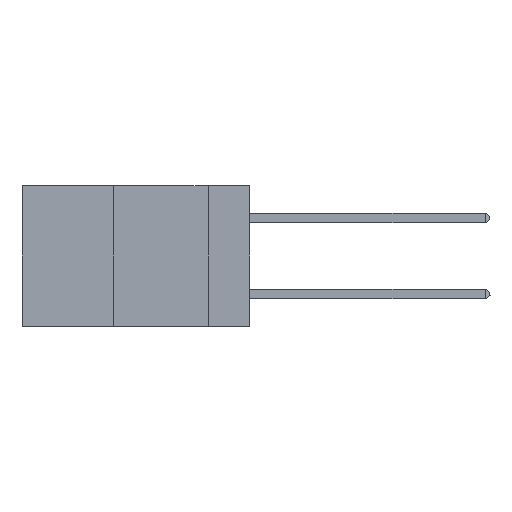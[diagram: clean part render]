
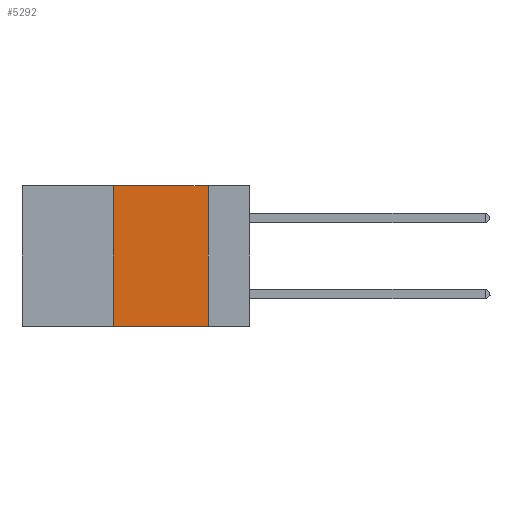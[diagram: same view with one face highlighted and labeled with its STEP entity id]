
A CAD part, left-side view. The second image highlights one B-rep face of the part: STEP entity #5292.
In plain terms, the highlighted planar face has unit normal (-1, 0, 0).
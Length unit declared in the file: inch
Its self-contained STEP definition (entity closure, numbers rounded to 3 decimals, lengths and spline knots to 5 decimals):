
#268 = CARTESIAN_POINT ( 'NONE',  ( 0., 0.36, 0. ) ) ;
#1010 = LINE ( 'NONE', #16282, #7445 ) ;
#1446 = VECTOR ( 'NONE', #27344, 39.37008 ) ;
#1500 = EDGE_CURVE ( 'NONE', #24219, #27783, #1010, .T. ) ;
#2094 = LINE ( 'NONE', #18200, #26129 ) ;
#2133 = CARTESIAN_POINT ( 'NONE',  ( 0., 0.36, 0. ) ) ;
#3128 = ORIENTED_EDGE ( 'NONE', *, *, #10522, .F. ) ;
#5292 = ADVANCED_FACE ( 'NONE', ( #23066 ), #11940, .F. ) ;
#7445 = VECTOR ( 'NONE', #11656, 39.37008 ) ;
#9451 = LINE ( 'NONE', #2133, #1446 ) ;
#10522 = EDGE_CURVE ( 'NONE', #24219, #12321, #9451, .T. ) ;
#11181 = VERTEX_POINT ( 'NONE', #14062 ) ;
#11422 = EDGE_LOOP ( 'NONE', ( #26074, #19471, #3128, #15519 ) ) ;
#11656 = DIRECTION ( 'NONE',  ( 0., -1., 0. ) ) ;
#11940 = PLANE ( 'NONE',  #20525 ) ;
#12321 = VERTEX_POINT ( 'NONE', #268 ) ;
#14044 = VECTOR ( 'NONE', #17275, 39.37008 ) ;
#14062 = CARTESIAN_POINT ( 'NONE',  ( 0., 0.11, 0. ) ) ;
#14481 = DIRECTION ( 'NONE',  ( 0., 0., -1. ) ) ;
#14801 = CARTESIAN_POINT ( 'NONE',  ( 0., 0.6, 0. ) ) ;
#15295 = CARTESIAN_POINT ( 'NONE',  ( 0., 0.11, -0.37 ) ) ;
#15519 = ORIENTED_EDGE ( 'NONE', *, *, #1500, .T. ) ;
#16282 = CARTESIAN_POINT ( 'NONE',  ( 0., 0.6, -0.37 ) ) ;
#17275 = DIRECTION ( 'NONE',  ( 0., -1., 0. ) ) ;
#18200 = CARTESIAN_POINT ( 'NONE',  ( 0., 0.11, 0. ) ) ;
#19471 = ORIENTED_EDGE ( 'NONE', *, *, #24892, .F. ) ;
#20525 = AXIS2_PLACEMENT_3D ( 'NONE', #14801, #29827, #14481 ) ;
#20664 = DIRECTION ( 'NONE',  ( 0., 0., -1. ) ) ;
#23066 = FACE_OUTER_BOUND ( 'NONE', #11422, .T. ) ;
#24219 = VERTEX_POINT ( 'NONE', #32777 ) ;
#24472 = EDGE_CURVE ( 'NONE', #11181, #27783, #2094, .T. ) ;
#24892 = EDGE_CURVE ( 'NONE', #12321, #11181, #27717, .T. ) ;
#25260 = CARTESIAN_POINT ( 'NONE',  ( 0., 0.6, 0. ) ) ;
#26074 = ORIENTED_EDGE ( 'NONE', *, *, #24472, .F. ) ;
#26129 = VECTOR ( 'NONE', #20664, 39.37008 ) ;
#27344 = DIRECTION ( 'NONE',  ( 0., 0., 1. ) ) ;
#27717 = LINE ( 'NONE', #25260, #14044 ) ;
#27783 = VERTEX_POINT ( 'NONE', #15295 ) ;
#29827 = DIRECTION ( 'NONE',  ( 1., 0., 0. ) ) ;
#32777 = CARTESIAN_POINT ( 'NONE',  ( 0., 0.36, -0.37 ) ) ;
